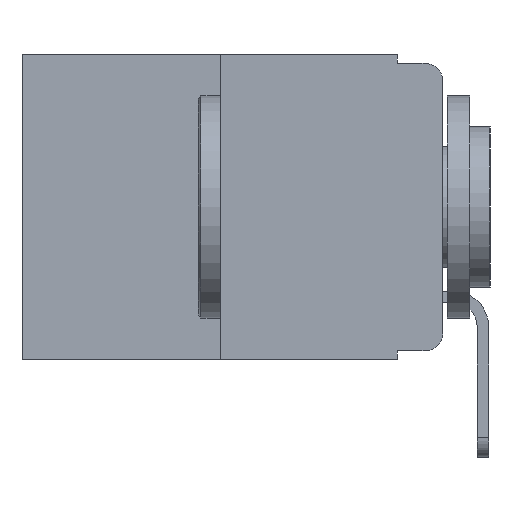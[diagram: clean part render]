
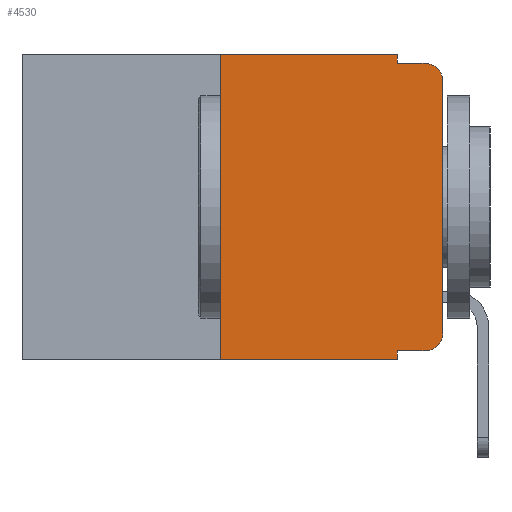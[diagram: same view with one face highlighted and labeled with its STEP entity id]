
A CAD part, left-side view. The second image highlights one B-rep face of the part: STEP entity #4530.
In plain terms, the highlighted planar face has unit normal (-1, 0, 0).
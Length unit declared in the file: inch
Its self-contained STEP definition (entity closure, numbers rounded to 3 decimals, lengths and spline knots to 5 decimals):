
#18 = EDGE_LOOP ( 'NONE', ( #4264, #6340, #8889, #9911, #12346, #2033, #2550, #10709, #10462, #12488 ) ) ;
#328 = CARTESIAN_POINT ( 'NONE',  ( 0., 0.473, 0. ) ) ;
#794 = VECTOR ( 'NONE', #16137, 39.37008 ) ;
#908 = CARTESIAN_POINT ( 'NONE',  ( 0., 0.473, 0. ) ) ;
#1033 = VERTEX_POINT ( 'NONE', #2999 ) ;
#1455 = VERTEX_POINT ( 'NONE', #14486 ) ;
#2033 = ORIENTED_EDGE ( 'NONE', *, *, #2991, .F. ) ;
#2401 = VECTOR ( 'NONE', #3962, 39.37008 ) ;
#2464 = VERTEX_POINT ( 'NONE', #6949 ) ;
#2496 = DIRECTION ( 'NONE',  ( -1., 0., 0. ) ) ;
#2550 = ORIENTED_EDGE ( 'NONE', *, *, #7555, .T. ) ;
#2958 = VERTEX_POINT ( 'NONE', #14050 ) ;
#2991 = EDGE_CURVE ( 'NONE', #1033, #10464, #5038, .T. ) ;
#2999 = CARTESIAN_POINT ( 'NONE',  ( 0., 0.25, -0.343 ) ) ;
#3001 = DIRECTION ( 'NONE',  ( -1., 0., 0. ) ) ;
#3053 = VERTEX_POINT ( 'NONE', #5129 ) ;
#3213 = EDGE_CURVE ( 'NONE', #8547, #3053, #16227, .T. ) ;
#3294 = CARTESIAN_POINT ( 'NONE',  ( 0., 0.25, 0. ) ) ;
#3302 = CARTESIAN_POINT ( 'NONE',  ( 0., 0., -0.03 ) ) ;
#3487 = EDGE_CURVE ( 'NONE', #5805, #1455, #9891, .T. ) ;
#3882 = VECTOR ( 'NONE', #9095, 39.37008 ) ;
#3962 = DIRECTION ( 'NONE',  ( 0., -1., 0. ) ) ;
#3999 = CARTESIAN_POINT ( 'NONE',  ( 0., 0.051, -0.333 ) ) ;
#4264 = ORIENTED_EDGE ( 'NONE', *, *, #13204, .T. ) ;
#4530 = ADVANCED_FACE ( 'NONE', ( #15744 ), #6048, .F. ) ;
#4647 = CARTESIAN_POINT ( 'NONE',  ( 0., 0.473, -0.343 ) ) ;
#4750 = DIRECTION ( 'NONE',  ( 0., 0., 1. ) ) ;
#4792 = CARTESIAN_POINT ( 'NONE',  ( 0., 0.051, 0. ) ) ;
#4924 = LINE ( 'NONE', #10065, #11465 ) ;
#5038 = LINE ( 'NONE', #5214, #5691 ) ;
#5129 = CARTESIAN_POINT ( 'NONE',  ( 0., 0.051, -0.343 ) ) ;
#5214 = CARTESIAN_POINT ( 'NONE',  ( 0., 0.25, 0. ) ) ;
#5232 = EDGE_CURVE ( 'NONE', #11102, #2464, #4924, .T. ) ;
#5691 = VECTOR ( 'NONE', #12626, 39.37008 ) ;
#5805 = VERTEX_POINT ( 'NONE', #11892 ) ;
#6048 = PLANE ( 'NONE',  #15483 ) ;
#6340 = ORIENTED_EDGE ( 'NONE', *, *, #6527, .T. ) ;
#6348 = LINE ( 'NONE', #16613, #6694 ) ;
#6527 = EDGE_CURVE ( 'NONE', #7430, #2958, #12039, .T. ) ;
#6660 = AXIS2_PLACEMENT_3D ( 'NONE', #11431, #2496, #7644 ) ;
#6694 = VECTOR ( 'NONE', #12670, 39.37008 ) ;
#6820 = CARTESIAN_POINT ( 'NONE',  ( 0., 0.051, -0.333 ) ) ;
#6886 = CARTESIAN_POINT ( 'NONE',  ( 0., 0.02, -0.03 ) ) ;
#6949 = CARTESIAN_POINT ( 'NONE',  ( 0., 0.051, -0.01 ) ) ;
#7318 = CARTESIAN_POINT ( 'NONE',  ( 0., 0.051, 0. ) ) ;
#7430 = VERTEX_POINT ( 'NONE', #3302 ) ;
#7555 = EDGE_CURVE ( 'NONE', #1033, #3053, #16179, .T. ) ;
#7644 = DIRECTION ( 'NONE',  ( 0., 0., -1. ) ) ;
#7832 = LINE ( 'NONE', #328, #2401 ) ;
#8547 = VERTEX_POINT ( 'NONE', #3999 ) ;
#8600 = EDGE_CURVE ( 'NONE', #2464, #2958, #6348, .T. ) ;
#8796 = DIRECTION ( 'NONE',  ( 0., 0., -1. ) ) ;
#8889 = ORIENTED_EDGE ( 'NONE', *, *, #8600, .F. ) ;
#9080 = AXIS2_PLACEMENT_3D ( 'NONE', #6886, #3001, #15715 ) ;
#9095 = DIRECTION ( 'NONE',  ( 0., -1., 0. ) ) ;
#9399 = EDGE_CURVE ( 'NONE', #10464, #11102, #7832, .T. ) ;
#9793 = DIRECTION ( 'NONE',  ( 0., -1., 0. ) ) ;
#9891 = CIRCLE ( 'NONE', #6660, 0.02 ) ;
#9911 = ORIENTED_EDGE ( 'NONE', *, *, #5232, .F. ) ;
#10065 = CARTESIAN_POINT ( 'NONE',  ( 0., 0.051, 0. ) ) ;
#10462 = ORIENTED_EDGE ( 'NONE', *, *, #15838, .T. ) ;
#10464 = VERTEX_POINT ( 'NONE', #3294 ) ;
#10615 = DIRECTION ( 'NONE',  ( 0., 0., -1. ) ) ;
#10709 = ORIENTED_EDGE ( 'NONE', *, *, #3213, .F. ) ;
#11102 = VERTEX_POINT ( 'NONE', #4792 ) ;
#11431 = CARTESIAN_POINT ( 'NONE',  ( 0., 0.02, -0.313 ) ) ;
#11465 = VECTOR ( 'NONE', #8796, 39.37008 ) ;
#11892 = CARTESIAN_POINT ( 'NONE',  ( 0., 0.02, -0.333 ) ) ;
#12039 = CIRCLE ( 'NONE', #9080, 0.02 ) ;
#12346 = ORIENTED_EDGE ( 'NONE', *, *, #9399, .F. ) ;
#12488 = ORIENTED_EDGE ( 'NONE', *, *, #3487, .T. ) ;
#12511 = CARTESIAN_POINT ( 'NONE',  ( 0., 0., 0. ) ) ;
#12626 = DIRECTION ( 'NONE',  ( 0., 0., 1. ) ) ;
#12670 = DIRECTION ( 'NONE',  ( 0., -1., 0. ) ) ;
#12751 = LINE ( 'NONE', #12511, #14850 ) ;
#13137 = LINE ( 'NONE', #6820, #3882 ) ;
#13204 = EDGE_CURVE ( 'NONE', #1455, #7430, #12751, .T. ) ;
#14050 = CARTESIAN_POINT ( 'NONE',  ( 0., 0.02, -0.01 ) ) ;
#14486 = CARTESIAN_POINT ( 'NONE',  ( 0., 0., -0.313 ) ) ;
#14699 = DIRECTION ( 'NONE',  ( 1., 0., 0. ) ) ;
#14850 = VECTOR ( 'NONE', #4750, 39.37008 ) ;
#15483 = AXIS2_PLACEMENT_3D ( 'NONE', #908, #14699, #10615 ) ;
#15715 = DIRECTION ( 'NONE',  ( 0., 0., -1. ) ) ;
#15744 = FACE_OUTER_BOUND ( 'NONE', #18, .T. ) ;
#15838 = EDGE_CURVE ( 'NONE', #8547, #5805, #13137, .T. ) ;
#16061 = VECTOR ( 'NONE', #9793, 39.37008 ) ;
#16137 = DIRECTION ( 'NONE',  ( 0., 0., -1. ) ) ;
#16179 = LINE ( 'NONE', #4647, #16061 ) ;
#16227 = LINE ( 'NONE', #7318, #794 ) ;
#16613 = CARTESIAN_POINT ( 'NONE',  ( 0., 0.051, -0.01 ) ) ;
